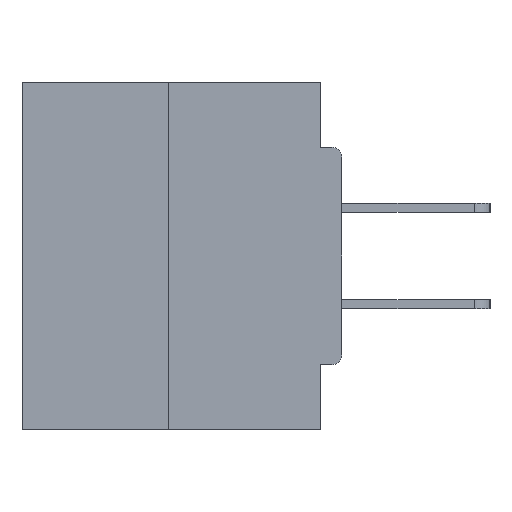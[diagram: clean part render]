
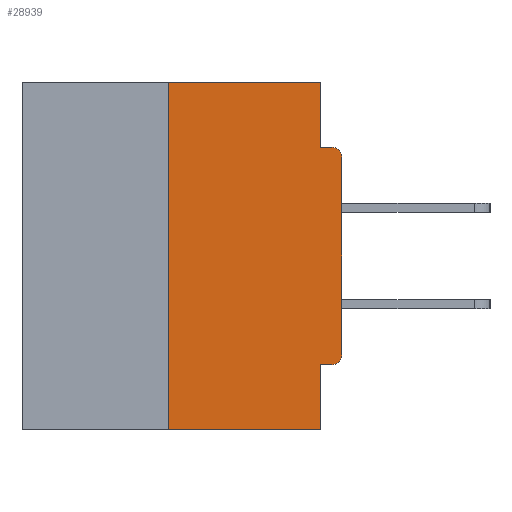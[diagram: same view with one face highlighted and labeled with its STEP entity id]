
A CAD part, left-side view. The second image highlights one B-rep face of the part: STEP entity #28939.
In plain terms, the highlighted planar face has unit normal (-1, 0, 0).
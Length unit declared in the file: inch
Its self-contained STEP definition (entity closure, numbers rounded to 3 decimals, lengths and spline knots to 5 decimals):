
#1352 = ORIENTED_EDGE ( 'NONE', *, *, #2247, .F. ) ;
#1415 = EDGE_LOOP ( 'NONE', ( #2668, #26664, #23356, #11667, #15343, #27125, #16208, #14436, #33916, #1352 ) ) ;
#1538 = VERTEX_POINT ( 'NONE', #19223 ) ;
#1980 = VECTOR ( 'NONE', #2067, 39.37008 ) ;
#2067 = DIRECTION ( 'NONE',  ( 0., 0., -1. ) ) ;
#2247 = EDGE_CURVE ( 'NONE', #25647, #32513, #31113, .T. ) ;
#2668 = ORIENTED_EDGE ( 'NONE', *, *, #4522, .F. ) ;
#2944 = CIRCLE ( 'NONE', #11679, 0.015 ) ;
#3216 = LINE ( 'NONE', #3424, #27915 ) ;
#3424 = CARTESIAN_POINT ( 'NONE',  ( 0., 0.031, -0.5 ) ) ;
#3566 = EDGE_CURVE ( 'NONE', #32513, #29172, #11885, .T. ) ;
#4522 = EDGE_CURVE ( 'NONE', #16765, #25647, #11797, .T. ) ;
#4900 = VERTEX_POINT ( 'NONE', #16014 ) ;
#5200 = DIRECTION ( 'NONE',  ( 0., -1., 0. ) ) ;
#5204 = DIRECTION ( 'NONE',  ( 0., -1., 0. ) ) ;
#5737 = CARTESIAN_POINT ( 'NONE',  ( 0., 0.015, -0.3915 ) ) ;
#6769 = VECTOR ( 'NONE', #16349, 39.37008 ) ;
#7357 = DIRECTION ( 'NONE',  ( 0., 0., 1. ) ) ;
#7495 = LINE ( 'NONE', #23581, #24546 ) ;
#7503 = AXIS2_PLACEMENT_3D ( 'NONE', #8907, #20207, #17448 ) ;
#8292 = DIRECTION ( 'NONE',  ( 0., 0., 1. ) ) ;
#8907 = CARTESIAN_POINT ( 'NONE',  ( 0., 0.015, -0.1085 ) ) ;
#10781 = CARTESIAN_POINT ( 'NONE',  ( 0., 0.031, 0. ) ) ;
#11013 = CARTESIAN_POINT ( 'NONE',  ( 0., 0.015, -0.0935 ) ) ;
#11014 = CARTESIAN_POINT ( 'NONE',  ( 0., 0.46, 0. ) ) ;
#11324 = CARTESIAN_POINT ( 'NONE',  ( 0., 0., 0. ) ) ;
#11667 = ORIENTED_EDGE ( 'NONE', *, *, #30067, .F. ) ;
#11679 = AXIS2_PLACEMENT_3D ( 'NONE', #5737, #28557, #31925 ) ;
#11797 = LINE ( 'NONE', #11014, #34647 ) ;
#11885 = LINE ( 'NONE', #33913, #25284 ) ;
#11917 = PLANE ( 'NONE',  #31230 ) ;
#12094 = DIRECTION ( 'NONE',  ( 0., -1., 0. ) ) ;
#12378 = LINE ( 'NONE', #11324, #19088 ) ;
#13166 = CARTESIAN_POINT ( 'NONE',  ( 0., 0.031, -0.5 ) ) ;
#13223 = EDGE_CURVE ( 'NONE', #23612, #34172, #12378, .T. ) ;
#14436 = ORIENTED_EDGE ( 'NONE', *, *, #28358, .T. ) ;
#15343 = ORIENTED_EDGE ( 'NONE', *, *, #18968, .F. ) ;
#16014 = CARTESIAN_POINT ( 'NONE',  ( 0., 0.031, -0.4065 ) ) ;
#16189 = CARTESIAN_POINT ( 'NONE',  ( 0., 0., -0.1085 ) ) ;
#16208 = ORIENTED_EDGE ( 'NONE', *, *, #13223, .T. ) ;
#16349 = DIRECTION ( 'NONE',  ( 0., 1., 0. ) ) ;
#16765 = VERTEX_POINT ( 'NONE', #17443 ) ;
#17443 = CARTESIAN_POINT ( 'NONE',  ( 0., 0.25, 0. ) ) ;
#17448 = DIRECTION ( 'NONE',  ( 0., 0., -1. ) ) ;
#18393 = CARTESIAN_POINT ( 'NONE',  ( 0., 0.25, 0. ) ) ;
#18689 = VECTOR ( 'NONE', #7357, 39.37008 ) ;
#18968 = EDGE_CURVE ( 'NONE', #22007, #4900, #27389, .T. ) ;
#19088 = VECTOR ( 'NONE', #8292, 39.37008 ) ;
#19145 = CIRCLE ( 'NONE', #7503, 0.015 ) ;
#19223 = CARTESIAN_POINT ( 'NONE',  ( 0., 0.25, -0.5 ) ) ;
#20161 = DIRECTION ( 'NONE',  ( 1., 0., 0. ) ) ;
#20207 = DIRECTION ( 'NONE',  ( -1., 0., 0. ) ) ;
#21079 = EDGE_CURVE ( 'NONE', #1538, #31051, #7495, .T. ) ;
#21217 = CARTESIAN_POINT ( 'NONE',  ( 0., 0.031, 0. ) ) ;
#22007 = VERTEX_POINT ( 'NONE', #22280 ) ;
#22100 = EDGE_CURVE ( 'NONE', #22007, #23612, #2944, .T. ) ;
#22280 = CARTESIAN_POINT ( 'NONE',  ( 0., 0.015, -0.4065 ) ) ;
#22996 = CARTESIAN_POINT ( 'NONE',  ( 0., 0.031, -0.0935 ) ) ;
#23356 = ORIENTED_EDGE ( 'NONE', *, *, #21079, .T. ) ;
#23524 = DIRECTION ( 'NONE',  ( 0., 0., -1. ) ) ;
#23581 = CARTESIAN_POINT ( 'NONE',  ( 0., 0.46, -0.5 ) ) ;
#23612 = VERTEX_POINT ( 'NONE', #30991 ) ;
#24546 = VECTOR ( 'NONE', #12094, 39.37008 ) ;
#25284 = VECTOR ( 'NONE', #5204, 39.37008 ) ;
#25647 = VERTEX_POINT ( 'NONE', #21217 ) ;
#26664 = ORIENTED_EDGE ( 'NONE', *, *, #34030, .F. ) ;
#27125 = ORIENTED_EDGE ( 'NONE', *, *, #22100, .T. ) ;
#27389 = LINE ( 'NONE', #33232, #6769 ) ;
#27915 = VECTOR ( 'NONE', #35039, 39.37008 ) ;
#28358 = EDGE_CURVE ( 'NONE', #34172, #29172, #19145, .T. ) ;
#28557 = DIRECTION ( 'NONE',  ( -1., 0., 0. ) ) ;
#28939 = ADVANCED_FACE ( 'NONE', ( #29847 ), #11917, .F. ) ;
#29172 = VERTEX_POINT ( 'NONE', #11013 ) ;
#29847 = FACE_OUTER_BOUND ( 'NONE', #1415, .T. ) ;
#30067 = EDGE_CURVE ( 'NONE', #4900, #31051, #3216, .T. ) ;
#30991 = CARTESIAN_POINT ( 'NONE',  ( 0., 0., -0.3915 ) ) ;
#31051 = VERTEX_POINT ( 'NONE', #13166 ) ;
#31113 = LINE ( 'NONE', #10781, #1980 ) ;
#31230 = AXIS2_PLACEMENT_3D ( 'NONE', #31914, #20161, #23524 ) ;
#31914 = CARTESIAN_POINT ( 'NONE',  ( 0., 0.46, 0. ) ) ;
#31925 = DIRECTION ( 'NONE',  ( 0., 0., -1. ) ) ;
#32513 = VERTEX_POINT ( 'NONE', #22996 ) ;
#32570 = LINE ( 'NONE', #18393, #18689 ) ;
#33232 = CARTESIAN_POINT ( 'NONE',  ( 0., 0., -0.4065 ) ) ;
#33913 = CARTESIAN_POINT ( 'NONE',  ( 0., 0., -0.0935 ) ) ;
#33916 = ORIENTED_EDGE ( 'NONE', *, *, #3566, .F. ) ;
#34030 = EDGE_CURVE ( 'NONE', #1538, #16765, #32570, .T. ) ;
#34172 = VERTEX_POINT ( 'NONE', #16189 ) ;
#34647 = VECTOR ( 'NONE', #5200, 39.37008 ) ;
#35039 = DIRECTION ( 'NONE',  ( 0., 0., -1. ) ) ;
